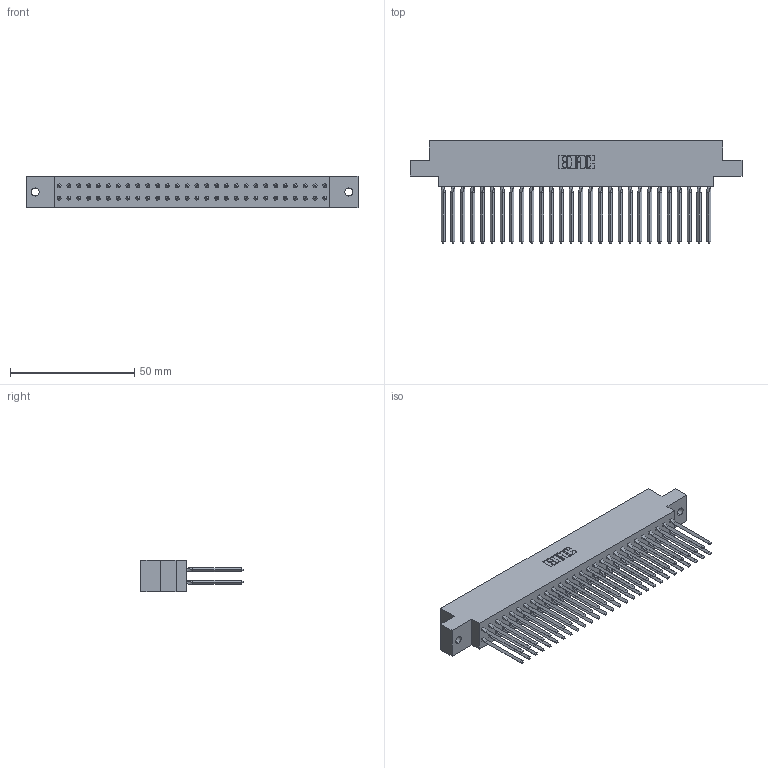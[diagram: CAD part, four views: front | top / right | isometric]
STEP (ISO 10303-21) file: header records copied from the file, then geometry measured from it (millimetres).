
FILE_DESCRIPTION (( 'STEP AP203' ), '1' );
FILE_NAME ('317-056-543-802.STEP', '2020-02-28T04:25:32', ( '' ), ( '' ), 'SwSTEP 2.0', 'SolidWorks 2016', '' );
FILE_SCHEMA (( 'CONFIG_CONTROL_DESIGN' ));
Length unit declared in the file: inch
Products named in the file (3): 317 Part_.144 Dia; 317-056-543-802; 317-290-001_543
Assembly tree (57 placements, depth 2):
  317-056-543-802
    317 Part_.144 Dia
    317-290-001_543  x56
Bounding box: 133.65 x 41.15 x 12.7 mm (x, y, z)
Volume: 22200.1 mm3; surface area: 32865.9 mm2
Topology: 57 solids, 57 shells, 5086 faces, 14107 edges, 9086 vertices
Faces by surface type: plane 4146, cylinder 716, bspline 224
Entity records: 42430 total; most frequent: CARTESIAN_POINT 7815, ORIENTED_EDGE 7314, DIRECTION 6103, EDGE_CURVE 3657, VECTOR 3401, LINE 3401, VERTEX_POINT 2431, AXIS2_PLACEMENT_3D 1351
